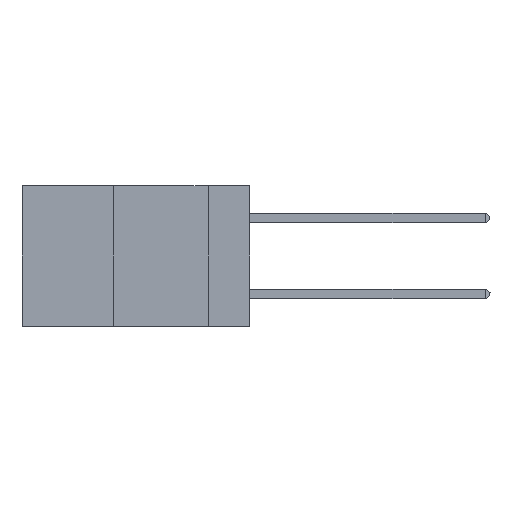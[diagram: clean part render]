
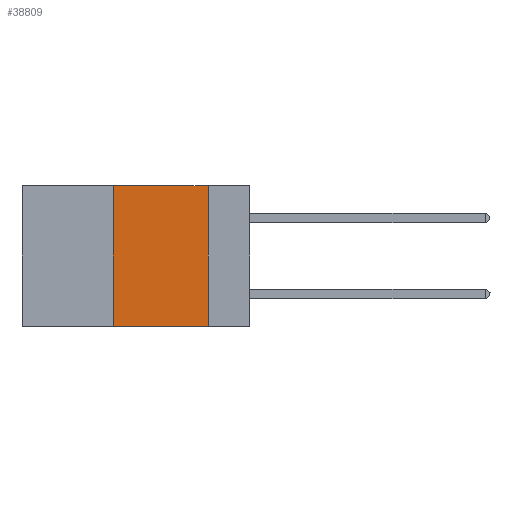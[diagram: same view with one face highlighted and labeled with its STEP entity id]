
A CAD part, left-side view. The second image highlights one B-rep face of the part: STEP entity #38809.
In plain terms, the highlighted planar face has unit normal (-1, 0, 0).
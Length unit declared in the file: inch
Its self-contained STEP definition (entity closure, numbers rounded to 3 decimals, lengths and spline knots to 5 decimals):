
#4290 = PLANE ( 'NONE',  #5989 ) ;
#4587 = CARTESIAN_POINT ( 'NONE',  ( 0., 0.36, -0.37 ) ) ;
#5989 = AXIS2_PLACEMENT_3D ( 'NONE', #7788, #11267, #35442 ) ;
#6080 = VERTEX_POINT ( 'NONE', #34386 ) ;
#6470 = LINE ( 'NONE', #22294, #30850 ) ;
#6933 = DIRECTION ( 'NONE',  ( 0., -1., 0. ) ) ;
#7094 = EDGE_CURVE ( 'NONE', #40527, #6080, #6470, .T. ) ;
#7756 = VECTOR ( 'NONE', #6933, 39.37008 ) ;
#7788 = CARTESIAN_POINT ( 'NONE',  ( 0., 0.6, 0. ) ) ;
#8316 = ORIENTED_EDGE ( 'NONE', *, *, #7094, .F. ) ;
#9166 = EDGE_LOOP ( 'NONE', ( #14279, #8316, #17532, #11574 ) ) ;
#10290 = VERTEX_POINT ( 'NONE', #4587 ) ;
#10756 = CARTESIAN_POINT ( 'NONE',  ( 0., 0.36, 0. ) ) ;
#11267 = DIRECTION ( 'NONE',  ( 1., 0., 0. ) ) ;
#11424 = EDGE_CURVE ( 'NONE', #10290, #12558, #18059, .T. ) ;
#11574 = ORIENTED_EDGE ( 'NONE', *, *, #11424, .T. ) ;
#11606 = DIRECTION ( 'NONE',  ( 0., 0., -1. ) ) ;
#11686 = EDGE_CURVE ( 'NONE', #6080, #12558, #33714, .T. ) ;
#12558 = VERTEX_POINT ( 'NONE', #26425 ) ;
#14279 = ORIENTED_EDGE ( 'NONE', *, *, #11686, .F. ) ;
#16964 = CARTESIAN_POINT ( 'NONE',  ( 0., 0.36, 0. ) ) ;
#17532 = ORIENTED_EDGE ( 'NONE', *, *, #30857, .F. ) ;
#18059 = LINE ( 'NONE', #20761, #7756 ) ;
#20761 = CARTESIAN_POINT ( 'NONE',  ( 0., 0.6, -0.37 ) ) ;
#21959 = CARTESIAN_POINT ( 'NONE',  ( 0., 0.11, 0. ) ) ;
#22294 = CARTESIAN_POINT ( 'NONE',  ( 0., 0.6, 0. ) ) ;
#24562 = VECTOR ( 'NONE', #11606, 39.37008 ) ;
#25766 = DIRECTION ( 'NONE',  ( 0., -1., 0. ) ) ;
#26425 = CARTESIAN_POINT ( 'NONE',  ( 0., 0.11, -0.37 ) ) ;
#29500 = VECTOR ( 'NONE', #41070, 39.37008 ) ;
#29919 = FACE_OUTER_BOUND ( 'NONE', #9166, .T. ) ;
#30850 = VECTOR ( 'NONE', #25766, 39.37008 ) ;
#30857 = EDGE_CURVE ( 'NONE', #10290, #40527, #37545, .T. ) ;
#33714 = LINE ( 'NONE', #21959, #24562 ) ;
#34386 = CARTESIAN_POINT ( 'NONE',  ( 0., 0.11, 0. ) ) ;
#35442 = DIRECTION ( 'NONE',  ( 0., 0., -1. ) ) ;
#37545 = LINE ( 'NONE', #16964, #29500 ) ;
#38809 = ADVANCED_FACE ( 'NONE', ( #29919 ), #4290, .F. ) ;
#40527 = VERTEX_POINT ( 'NONE', #10756 ) ;
#41070 = DIRECTION ( 'NONE',  ( 0., 0., 1. ) ) ;
